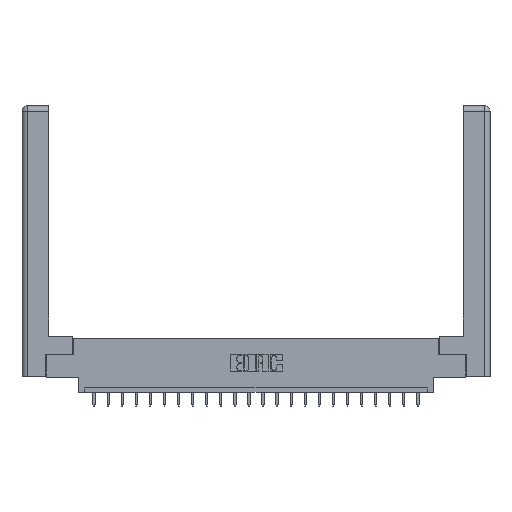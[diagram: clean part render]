
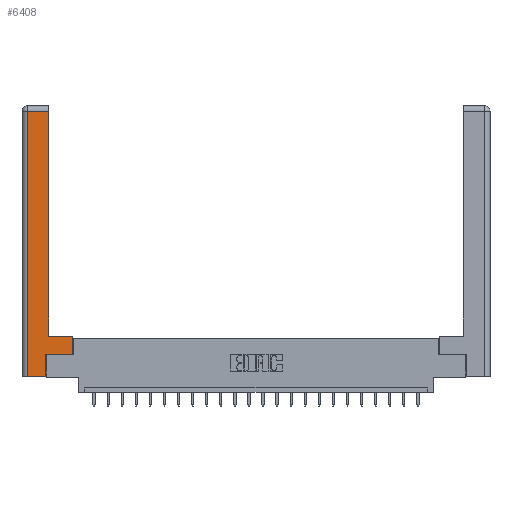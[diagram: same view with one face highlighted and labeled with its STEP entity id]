
A CAD part, top view. The second image highlights one B-rep face of the part: STEP entity #6408.
In plain terms, the highlighted planar face has unit normal (0, 0, 1).
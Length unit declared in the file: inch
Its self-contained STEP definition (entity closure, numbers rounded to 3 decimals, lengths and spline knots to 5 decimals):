
#924 = VECTOR ( 'NONE', #9653, 39.37008 ) ;
#925 = VERTEX_POINT ( 'NONE', #22572 ) ;
#1322 = CARTESIAN_POINT ( 'NONE',  ( 0.565, 0.245, 0. ) ) ;
#1442 = LINE ( 'NONE', #2760, #19453 ) ;
#2599 = LINE ( 'NONE', #8144, #7585 ) ;
#2760 = CARTESIAN_POINT ( 'NONE',  ( 0.295, 3., 0. ) ) ;
#3288 = VERTEX_POINT ( 'NONE', #3832 ) ;
#3458 = CARTESIAN_POINT ( 'NONE',  ( 0., 0., 0. ) ) ;
#3543 = DIRECTION ( 'NONE',  ( -1., 0., 0. ) ) ;
#3549 = VECTOR ( 'NONE', #7390, 39.37008 ) ;
#3620 = CARTESIAN_POINT ( 'NONE',  ( 0.565, 0.245, 0. ) ) ;
#3716 = CARTESIAN_POINT ( 'NONE',  ( 0.0615, 0., 0. ) ) ;
#3731 = EDGE_LOOP ( 'NONE', ( #18866, #20399, #17361, #7444, #15381, #21096, #16354, #21106 ) ) ;
#3832 = CARTESIAN_POINT ( 'NONE',  ( 0.0615, 2.94, 0. ) ) ;
#3865 = DIRECTION ( 'NONE',  ( 1., 0., 0. ) ) ;
#3935 = CARTESIAN_POINT ( 'NONE',  ( 0.265, 0.245, 0. ) ) ;
#5469 = VERTEX_POINT ( 'NONE', #14928 ) ;
#6066 = LINE ( 'NONE', #3716, #3549 ) ;
#6342 = EDGE_CURVE ( 'NONE', #13260, #5469, #12315, .T. ) ;
#6347 = DIRECTION ( 'NONE',  ( 0., 1., 0. ) ) ;
#6408 = ADVANCED_FACE ( 'NONE', ( #6533 ), #19414, .F. ) ;
#6521 = CARTESIAN_POINT ( 'NONE',  ( 0.265, 0.245, 0. ) ) ;
#6533 = FACE_OUTER_BOUND ( 'NONE', #3731, .T. ) ;
#7272 = LINE ( 'NONE', #3935, #19990 ) ;
#7390 = DIRECTION ( 'NONE',  ( 0., -1., 0. ) ) ;
#7444 = ORIENTED_EDGE ( 'NONE', *, *, #19763, .T. ) ;
#7541 = LINE ( 'NONE', #13173, #11673 ) ;
#7585 = VECTOR ( 'NONE', #20520, 39.37008 ) ;
#7596 = DIRECTION ( 'NONE',  ( 0., 1., 0. ) ) ;
#7933 = EDGE_CURVE ( 'NONE', #925, #10773, #7272, .T. ) ;
#8144 = CARTESIAN_POINT ( 'NONE',  ( 0.265, 0., 0. ) ) ;
#8504 = EDGE_CURVE ( 'NONE', #10773, #13260, #21620, .T. ) ;
#8832 = CARTESIAN_POINT ( 'NONE',  ( 0.295, 0.45, 0. ) ) ;
#9465 = CARTESIAN_POINT ( 'NONE',  ( 0.0615, 0., 0. ) ) ;
#9525 = LINE ( 'NONE', #15039, #924 ) ;
#9653 = DIRECTION ( 'NONE',  ( -1., 0., 0. ) ) ;
#9887 = CARTESIAN_POINT ( 'NONE',  ( 0.295, 2.94, 0. ) ) ;
#10011 = EDGE_CURVE ( 'NONE', #16860, #21505, #1442, .T. ) ;
#10773 = VERTEX_POINT ( 'NONE', #6521 ) ;
#11253 = DIRECTION ( 'NONE',  ( -1., 0., 0. ) ) ;
#11314 = EDGE_CURVE ( 'NONE', #5469, #16860, #7541, .T. ) ;
#11641 = VECTOR ( 'NONE', #3865, 39.37008 ) ;
#11673 = VECTOR ( 'NONE', #11253, 39.37008 ) ;
#12315 = LINE ( 'NONE', #20955, #15938 ) ;
#13001 = EDGE_CURVE ( 'NONE', #3288, #19421, #6066, .T. ) ;
#13173 = CARTESIAN_POINT ( 'NONE',  ( 0.295, 0.45, 0. ) ) ;
#13260 = VERTEX_POINT ( 'NONE', #1322 ) ;
#14142 = DIRECTION ( 'NONE',  ( 0., 0., -1. ) ) ;
#14928 = CARTESIAN_POINT ( 'NONE',  ( 0.565, 0.45, 0. ) ) ;
#15039 = CARTESIAN_POINT ( 'NONE',  ( 0.0615, 2.94, 0. ) ) ;
#15363 = EDGE_CURVE ( 'NONE', #21505, #3288, #9525, .T. ) ;
#15381 = ORIENTED_EDGE ( 'NONE', *, *, #7933, .T. ) ;
#15558 = AXIS2_PLACEMENT_3D ( 'NONE', #3458, #14142, #3543 ) ;
#15938 = VECTOR ( 'NONE', #20730, 39.37008 ) ;
#16354 = ORIENTED_EDGE ( 'NONE', *, *, #6342, .T. ) ;
#16860 = VERTEX_POINT ( 'NONE', #8832 ) ;
#17361 = ORIENTED_EDGE ( 'NONE', *, *, #13001, .T. ) ;
#18866 = ORIENTED_EDGE ( 'NONE', *, *, #10011, .T. ) ;
#19414 = PLANE ( 'NONE',  #15558 ) ;
#19421 = VERTEX_POINT ( 'NONE', #9465 ) ;
#19453 = VECTOR ( 'NONE', #6347, 39.37008 ) ;
#19763 = EDGE_CURVE ( 'NONE', #19421, #925, #2599, .T. ) ;
#19990 = VECTOR ( 'NONE', #7596, 39.37008 ) ;
#20399 = ORIENTED_EDGE ( 'NONE', *, *, #15363, .T. ) ;
#20520 = DIRECTION ( 'NONE',  ( 1., 0., 0. ) ) ;
#20730 = DIRECTION ( 'NONE',  ( 0., 1., 0. ) ) ;
#20955 = CARTESIAN_POINT ( 'NONE',  ( 0.565, 0.45, 0. ) ) ;
#21096 = ORIENTED_EDGE ( 'NONE', *, *, #8504, .T. ) ;
#21106 = ORIENTED_EDGE ( 'NONE', *, *, #11314, .T. ) ;
#21505 = VERTEX_POINT ( 'NONE', #9887 ) ;
#21620 = LINE ( 'NONE', #3620, #11641 ) ;
#22572 = CARTESIAN_POINT ( 'NONE',  ( 0.265, 0., 0. ) ) ;
